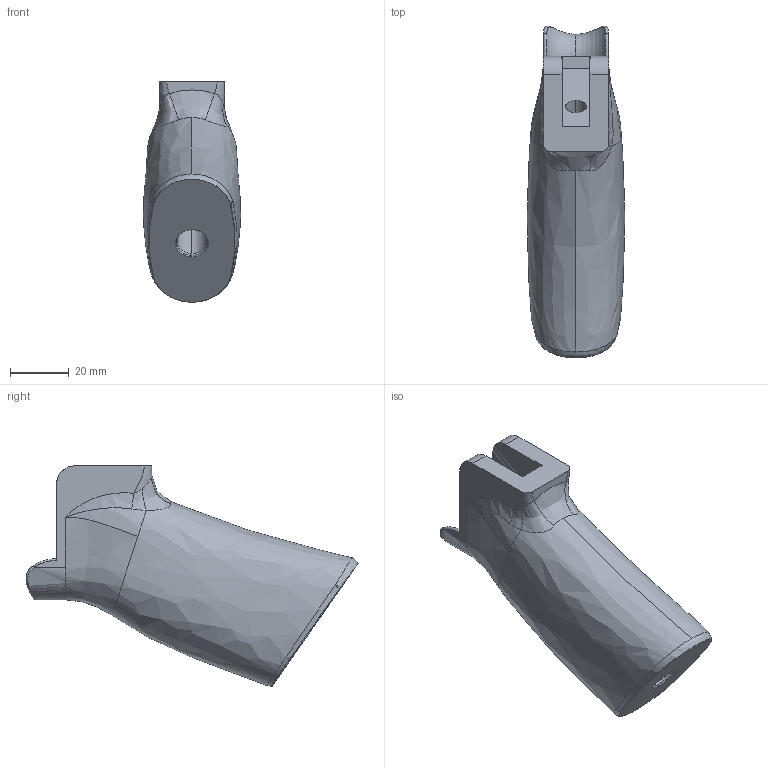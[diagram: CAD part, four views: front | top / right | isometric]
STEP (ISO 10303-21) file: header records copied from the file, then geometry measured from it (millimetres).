
FILE_DESCRIPTION (( 'STEP AP203' ), '1' );
FILE_NAME ('Grip V3.1 NT.STEP', '2022-05-14T17:19:44', ( '' ), ( '' ), 'SwSTEP 2.0', 'SolidWorks 2021', '' );
FILE_SCHEMA (( 'CONFIG_CONTROL_DESIGN' ));
Length unit declared in the file: inch
Products named in the file (1): Grip V3.1 NT
Bounding box: 33.2 x 113.29 x 75.17 mm (x, y, z)
Volume: 105537.5 mm3; surface area: 18741.3 mm2
Topology: 1 solids, 1 shells, 67 faces, 185 edges, 119 vertices
Faces by surface type: bspline 35, plane 14, cylinder 12, torus 6
Entity records: 7427 total; most frequent: CARTESIAN_POINT 5947, ORIENTED_EDGE 362, DIRECTION 188, EDGE_CURVE 181, VERTEX_POINT 119, B_SPLINE_CURVE_WITH_KNOTS 90, EDGE_LOOP 72, AXIS2_PLACEMENT_3D 72
